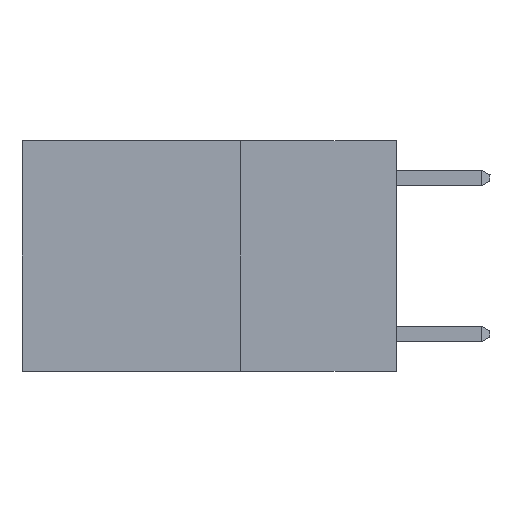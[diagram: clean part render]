
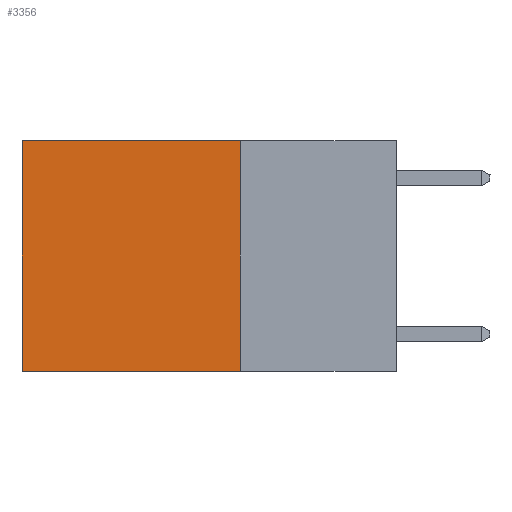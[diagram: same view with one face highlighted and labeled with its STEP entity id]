
A CAD part, left-side view. The second image highlights one B-rep face of the part: STEP entity #3356.
In plain terms, the highlighted planar face has unit normal (-1, 0, 0).
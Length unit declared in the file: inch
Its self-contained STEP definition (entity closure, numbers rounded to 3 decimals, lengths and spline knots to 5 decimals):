
#328 = PLANE ( 'NONE',  #2714 ) ;
#483 = FACE_OUTER_BOUND ( 'NONE', #8681, .T. ) ;
#1063 = CARTESIAN_POINT ( 'NONE',  ( 0.2625, 0.25, -0.37 ) ) ;
#1182 = DIRECTION ( 'NONE',  ( 0., 0., -1. ) ) ;
#1303 = LINE ( 'NONE', #10357, #5845 ) ;
#1335 = VERTEX_POINT ( 'NONE', #1063 ) ;
#1914 = ORIENTED_EDGE ( 'NONE', *, *, #8726, .F. ) ;
#2048 = VECTOR ( 'NONE', #8838, 39.37008 ) ;
#2714 = AXIS2_PLACEMENT_3D ( 'NONE', #9699, #6549, #1182 ) ;
#3071 = DIRECTION ( 'NONE',  ( 0., 1., 0. ) ) ;
#3318 = EDGE_CURVE ( 'NONE', #7015, #9710, #1303, .T. ) ;
#3356 = ADVANCED_FACE ( 'NONE', ( #483 ), #328, .F. ) ;
#4002 = CARTESIAN_POINT ( 'NONE',  ( 0.2625, 0.25, -0.37 ) ) ;
#4600 = DIRECTION ( 'NONE',  ( 0., 0., -1. ) ) ;
#4742 = CARTESIAN_POINT ( 'NONE',  ( 0.2625, 0.25, 0. ) ) ;
#4969 = EDGE_CURVE ( 'NONE', #1335, #9710, #10793, .T. ) ;
#5091 = CARTESIAN_POINT ( 'NONE',  ( 0.2625, 0.6, 0. ) ) ;
#5736 = EDGE_CURVE ( 'NONE', #10178, #7015, #9045, .T. ) ;
#5845 = VECTOR ( 'NONE', #4600, 39.37008 ) ;
#6095 = CARTESIAN_POINT ( 'NONE',  ( 0.2625, 0.25, 0. ) ) ;
#6549 = DIRECTION ( 'NONE',  ( 1., 0., 0. ) ) ;
#6611 = ORIENTED_EDGE ( 'NONE', *, *, #5736, .T. ) ;
#6960 = LINE ( 'NONE', #9607, #2048 ) ;
#7015 = VERTEX_POINT ( 'NONE', #5091 ) ;
#8248 = ORIENTED_EDGE ( 'NONE', *, *, #4969, .F. ) ;
#8538 = VECTOR ( 'NONE', #3071, 39.37008 ) ;
#8681 = EDGE_LOOP ( 'NONE', ( #10061, #8248, #1914, #6611 ) ) ;
#8726 = EDGE_CURVE ( 'NONE', #10178, #1335, #6960, .T. ) ;
#8838 = DIRECTION ( 'NONE',  ( 0., 0., -1. ) ) ;
#8997 = CARTESIAN_POINT ( 'NONE',  ( 0.2625, 0.6, -0.37 ) ) ;
#9045 = LINE ( 'NONE', #4742, #10798 ) ;
#9607 = CARTESIAN_POINT ( 'NONE',  ( 0.2625, 0.25, 0. ) ) ;
#9637 = DIRECTION ( 'NONE',  ( 0., 1., 0. ) ) ;
#9699 = CARTESIAN_POINT ( 'NONE',  ( 0.2625, 0.25, 0. ) ) ;
#9710 = VERTEX_POINT ( 'NONE', #8997 ) ;
#10061 = ORIENTED_EDGE ( 'NONE', *, *, #3318, .T. ) ;
#10178 = VERTEX_POINT ( 'NONE', #6095 ) ;
#10357 = CARTESIAN_POINT ( 'NONE',  ( 0.2625, 0.6, 0. ) ) ;
#10793 = LINE ( 'NONE', #4002, #8538 ) ;
#10798 = VECTOR ( 'NONE', #9637, 39.37008 ) ;
